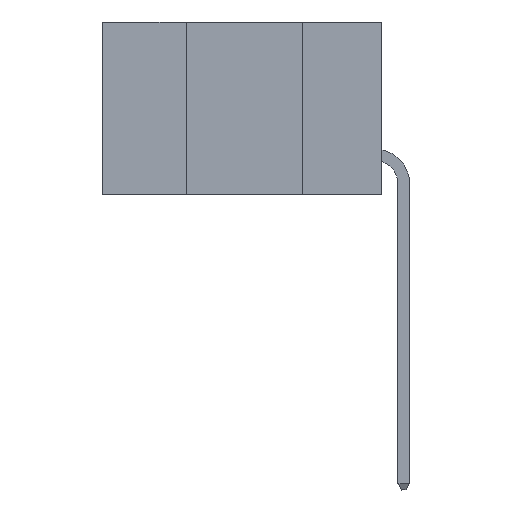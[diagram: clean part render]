
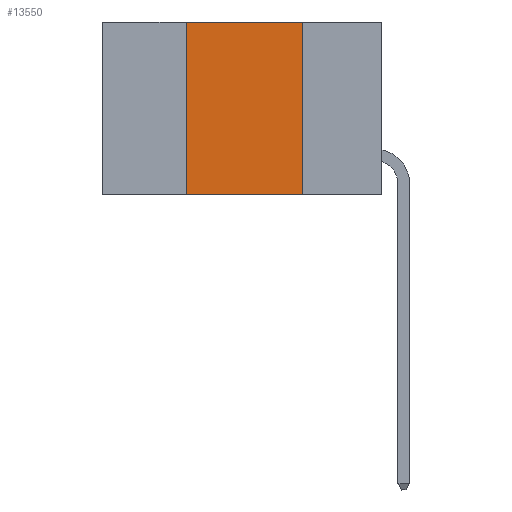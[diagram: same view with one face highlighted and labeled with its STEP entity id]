
A CAD part, left-side view. The second image highlights one B-rep face of the part: STEP entity #13550.
In plain terms, the highlighted planar face has unit normal (-1, 0, 0).
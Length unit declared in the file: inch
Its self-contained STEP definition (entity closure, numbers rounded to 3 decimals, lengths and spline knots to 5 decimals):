
#422 = EDGE_CURVE ( 'NONE', #17431, #15992, #4443, .T. ) ;
#605 = CARTESIAN_POINT ( 'NONE',  ( 0., 0.42, 0. ) ) ;
#916 = FACE_OUTER_BOUND ( 'NONE', #3266, .T. ) ;
#2394 = ORIENTED_EDGE ( 'NONE', *, *, #13331, .F. ) ;
#2652 = DIRECTION ( 'NONE',  ( 0., -1., 0. ) ) ;
#2937 = VECTOR ( 'NONE', #15813, 39.37008 ) ;
#2974 = ORIENTED_EDGE ( 'NONE', *, *, #422, .T. ) ;
#3266 = EDGE_LOOP ( 'NONE', ( #2394, #16039, #18473, #2974 ) ) ;
#4197 = VERTEX_POINT ( 'NONE', #605 ) ;
#4443 = LINE ( 'NONE', #10383, #8081 ) ;
#5347 = LINE ( 'NONE', #7841, #11895 ) ;
#7801 = EDGE_CURVE ( 'NONE', #4197, #14484, #15816, .T. ) ;
#7841 = CARTESIAN_POINT ( 'NONE',  ( 0., 0.17, 0. ) ) ;
#7975 = PLANE ( 'NONE',  #17557 ) ;
#8081 = VECTOR ( 'NONE', #2652, 39.37008 ) ;
#9587 = CARTESIAN_POINT ( 'NONE',  ( 0., 0.42, 0. ) ) ;
#10383 = CARTESIAN_POINT ( 'NONE',  ( 0., 0.6, -0.37 ) ) ;
#11692 = EDGE_CURVE ( 'NONE', #17431, #4197, #17258, .T. ) ;
#11895 = VECTOR ( 'NONE', #18483, 39.37008 ) ;
#12908 = CARTESIAN_POINT ( 'NONE',  ( 0., 0.6, 0. ) ) ;
#13331 = EDGE_CURVE ( 'NONE', #14484, #15992, #5347, .T. ) ;
#13411 = CARTESIAN_POINT ( 'NONE',  ( 0., 0.42, -0.37 ) ) ;
#13550 = ADVANCED_FACE ( 'NONE', ( #916 ), #7975, .F. ) ;
#14393 = CARTESIAN_POINT ( 'NONE',  ( 0., 0.6, 0. ) ) ;
#14484 = VERTEX_POINT ( 'NONE', #19947 ) ;
#15588 = VECTOR ( 'NONE', #15725, 39.37008 ) ;
#15725 = DIRECTION ( 'NONE',  ( 0., 0., 1. ) ) ;
#15735 = DIRECTION ( 'NONE',  ( 1., 0., 0. ) ) ;
#15813 = DIRECTION ( 'NONE',  ( 0., -1., 0. ) ) ;
#15816 = LINE ( 'NONE', #14393, #2937 ) ;
#15992 = VERTEX_POINT ( 'NONE', #17955 ) ;
#16039 = ORIENTED_EDGE ( 'NONE', *, *, #7801, .F. ) ;
#17258 = LINE ( 'NONE', #9587, #15588 ) ;
#17431 = VERTEX_POINT ( 'NONE', #13411 ) ;
#17557 = AXIS2_PLACEMENT_3D ( 'NONE', #12908, #15735, #18895 ) ;
#17955 = CARTESIAN_POINT ( 'NONE',  ( 0., 0.17, -0.37 ) ) ;
#18473 = ORIENTED_EDGE ( 'NONE', *, *, #11692, .F. ) ;
#18483 = DIRECTION ( 'NONE',  ( 0., 0., -1. ) ) ;
#18895 = DIRECTION ( 'NONE',  ( 0., 0., -1. ) ) ;
#19947 = CARTESIAN_POINT ( 'NONE',  ( 0., 0.17, 0. ) ) ;
